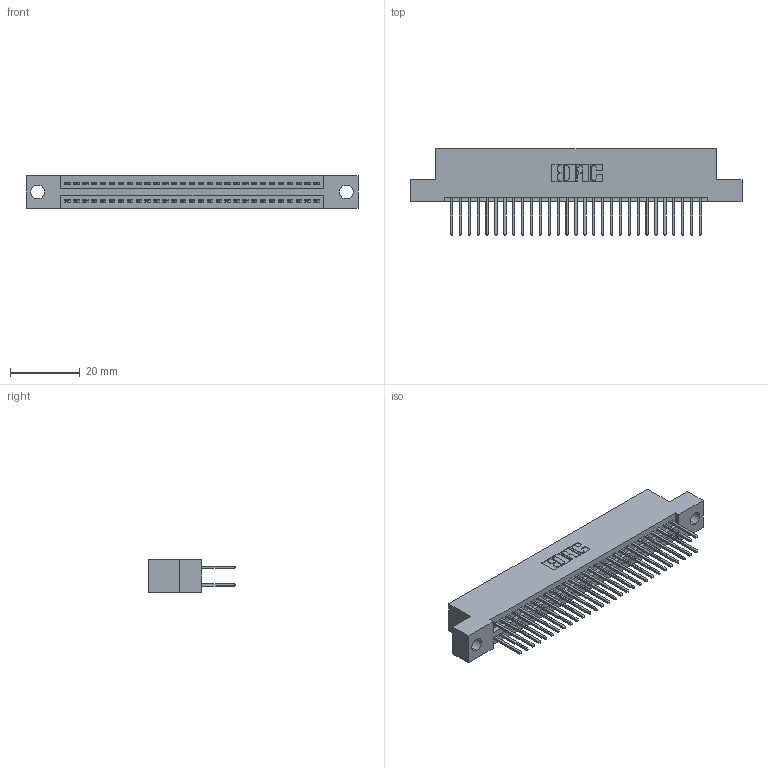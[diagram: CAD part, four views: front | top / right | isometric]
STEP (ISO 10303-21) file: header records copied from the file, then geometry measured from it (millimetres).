
FILE_DESCRIPTION (( 'STEP AP203' ), '1' );
FILE_NAME ('395-058-523-204.STEP', '2021-06-17T01:30:20', ( '' ), ( '' ), 'SwSTEP 2.0', 'SolidWorks 2020', '' );
FILE_SCHEMA (( 'CONFIG_CONTROL_DESIGN' ));
Length unit declared in the file: inch
Products named in the file (3): 345 Part_Flush Mounting Lugs - 0.156 Dia-TI; 345-292-001_345-293-123; 395-058-523-204
Assembly tree (59 placements, depth 2):
  395-058-523-204
    345 Part_Flush Mounting Lugs - 0.156 Dia-TI
    345-292-001_345-293-123  x58
Bounding box: 94.87 x 24.82 x 9.4 mm (x, y, z)
Volume: 9107.9 mm3; surface area: 13596.1 mm2
Topology: 59 solids, 59 shells, 3040 faces, 9019 edges, 5934 vertices
Faces by surface type: plane 2008, cylinder 1032
Entity records: 24941 total; most frequent: CARTESIAN_POINT 4198, ORIENTED_EDGE 4130, DIRECTION 3717, EDGE_CURVE 2065, VECTOR 1817, LINE 1817, VERTEX_POINT 1374, AXIS2_PLACEMENT_3D 950
